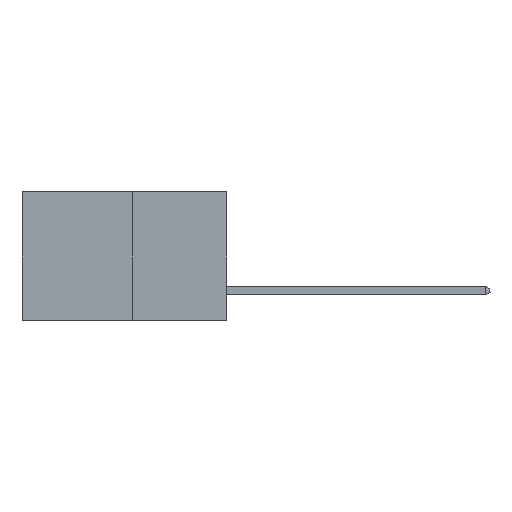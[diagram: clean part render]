
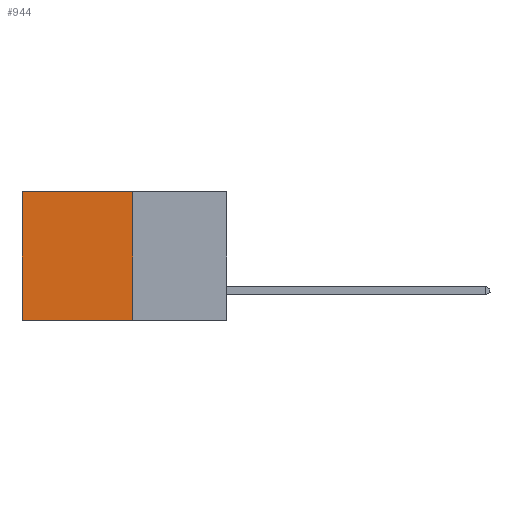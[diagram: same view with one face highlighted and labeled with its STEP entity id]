
A CAD part, left-side view. The second image highlights one B-rep face of the part: STEP entity #944.
In plain terms, the highlighted planar face has unit normal (-1, 0, 0).
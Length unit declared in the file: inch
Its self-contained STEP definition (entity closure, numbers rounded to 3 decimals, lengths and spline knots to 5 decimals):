
#236 = LINE ( 'NONE', #2878, #6071 ) ;
#774 = ORIENTED_EDGE ( 'NONE', *, *, #10631, .F. ) ;
#944 = ADVANCED_FACE ( 'NONE', ( #7819 ), #6522, .F. ) ;
#998 = LINE ( 'NONE', #2101, #6805 ) ;
#1644 = DIRECTION ( 'NONE',  ( 1., 0., 0. ) ) ;
#1808 = CARTESIAN_POINT ( 'NONE',  ( 0.277, 0.27, -0.37 ) ) ;
#2101 = CARTESIAN_POINT ( 'NONE',  ( 0.277, 0.59, -0.37 ) ) ;
#2204 = DIRECTION ( 'NONE',  ( 0., 1., 0. ) ) ;
#2878 = CARTESIAN_POINT ( 'NONE',  ( 0.277, 0.27, -0.37 ) ) ;
#3336 = VERTEX_POINT ( 'NONE', #12824 ) ;
#4765 = EDGE_LOOP ( 'NONE', ( #13931, #13468, #774, #6371 ) ) ;
#5117 = LINE ( 'NONE', #9065, #13859 ) ;
#6071 = VECTOR ( 'NONE', #11846, 39.37008 ) ;
#6371 = ORIENTED_EDGE ( 'NONE', *, *, #11411, .T. ) ;
#6400 = VECTOR ( 'NONE', #14178, 39.37008 ) ;
#6522 = PLANE ( 'NONE',  #10469 ) ;
#6805 = VECTOR ( 'NONE', #7885, 39.37008 ) ;
#7027 = VERTEX_POINT ( 'NONE', #10007 ) ;
#7549 = EDGE_CURVE ( 'NONE', #7027, #10669, #998, .T. ) ;
#7819 = FACE_OUTER_BOUND ( 'NONE', #4765, .T. ) ;
#7885 = DIRECTION ( 'NONE',  ( 0., 0., -1. ) ) ;
#8661 = CARTESIAN_POINT ( 'NONE',  ( 0.277, 0.59, -0.37 ) ) ;
#9065 = CARTESIAN_POINT ( 'NONE',  ( 0.277, 0.27, -0.37 ) ) ;
#9594 = EDGE_CURVE ( 'NONE', #3336, #10669, #5117, .T. ) ;
#9940 = DIRECTION ( 'NONE',  ( 0., 0., -1. ) ) ;
#10007 = CARTESIAN_POINT ( 'NONE',  ( 0.277, 0.59, 0. ) ) ;
#10469 = AXIS2_PLACEMENT_3D ( 'NONE', #1808, #1644, #9940 ) ;
#10631 = EDGE_CURVE ( 'NONE', #12161, #3336, #236, .T. ) ;
#10669 = VERTEX_POINT ( 'NONE', #8661 ) ;
#11411 = EDGE_CURVE ( 'NONE', #12161, #7027, #12237, .T. ) ;
#11846 = DIRECTION ( 'NONE',  ( 0., 0., -1. ) ) ;
#12050 = CARTESIAN_POINT ( 'NONE',  ( 0.277, 0.27, 0. ) ) ;
#12161 = VERTEX_POINT ( 'NONE', #13511 ) ;
#12237 = LINE ( 'NONE', #12050, #6400 ) ;
#12824 = CARTESIAN_POINT ( 'NONE',  ( 0.277, 0.27, -0.37 ) ) ;
#13468 = ORIENTED_EDGE ( 'NONE', *, *, #9594, .F. ) ;
#13511 = CARTESIAN_POINT ( 'NONE',  ( 0.277, 0.27, 0. ) ) ;
#13859 = VECTOR ( 'NONE', #2204, 39.37008 ) ;
#13931 = ORIENTED_EDGE ( 'NONE', *, *, #7549, .T. ) ;
#14178 = DIRECTION ( 'NONE',  ( 0., 1., 0. ) ) ;
